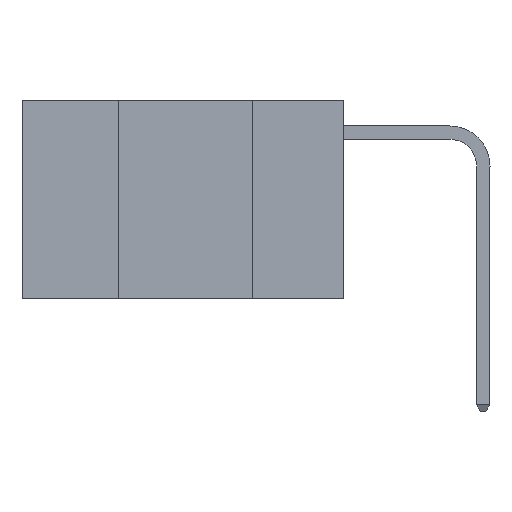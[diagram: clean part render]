
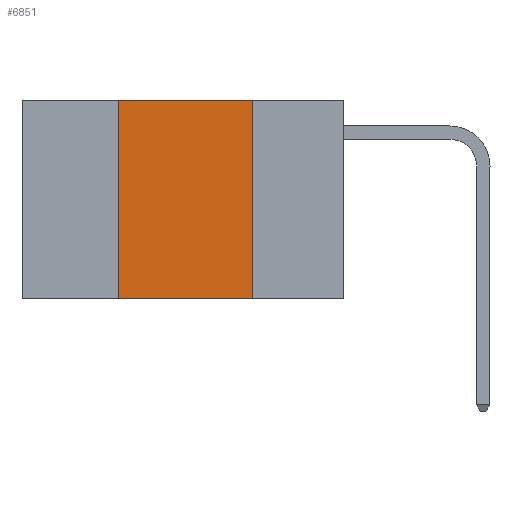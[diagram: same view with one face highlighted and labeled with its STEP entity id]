
A CAD part, left-side view. The second image highlights one B-rep face of the part: STEP entity #6851.
In plain terms, the highlighted planar face has unit normal (-1, 0, 0).
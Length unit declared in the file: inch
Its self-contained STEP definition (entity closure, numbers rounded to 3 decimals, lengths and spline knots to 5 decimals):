
#168 = VECTOR ( 'NONE', #7796, 39.37008 ) ;
#457 = CARTESIAN_POINT ( 'NONE',  ( 0., 0.17, 0. ) ) ;
#489 = ORIENTED_EDGE ( 'NONE', *, *, #13231, .F. ) ;
#883 = CARTESIAN_POINT ( 'NONE',  ( 0., 0.6, 0. ) ) ;
#902 = VERTEX_POINT ( 'NONE', #7395 ) ;
#962 = FACE_OUTER_BOUND ( 'NONE', #11207, .T. ) ;
#1337 = VECTOR ( 'NONE', #9512, 39.37008 ) ;
#1562 = VERTEX_POINT ( 'NONE', #9704 ) ;
#2855 = LINE ( 'NONE', #457, #9727 ) ;
#3279 = LINE ( 'NONE', #13469, #9341 ) ;
#3357 = VERTEX_POINT ( 'NONE', #3571 ) ;
#3571 = CARTESIAN_POINT ( 'NONE',  ( 0., 0.17, 0. ) ) ;
#3733 = DIRECTION ( 'NONE',  ( 0., -1., 0. ) ) ;
#5441 = CARTESIAN_POINT ( 'NONE',  ( 0., 0.42, 0. ) ) ;
#5551 = CARTESIAN_POINT ( 'NONE',  ( 0., 0.42, -0.37 ) ) ;
#6334 = DIRECTION ( 'NONE',  ( 0., 0., -1. ) ) ;
#6836 = LINE ( 'NONE', #5441, #168 ) ;
#6851 = ADVANCED_FACE ( 'NONE', ( #962 ), #11250, .F. ) ;
#7395 = CARTESIAN_POINT ( 'NONE',  ( 0., 0.42, 0. ) ) ;
#7500 = ORIENTED_EDGE ( 'NONE', *, *, #15976, .F. ) ;
#7796 = DIRECTION ( 'NONE',  ( 0., 0., 1. ) ) ;
#7878 = ORIENTED_EDGE ( 'NONE', *, *, #9794, .T. ) ;
#9135 = DIRECTION ( 'NONE',  ( 0., 0., -1. ) ) ;
#9341 = VECTOR ( 'NONE', #3733, 39.37008 ) ;
#9512 = DIRECTION ( 'NONE',  ( 0., -1., 0. ) ) ;
#9704 = CARTESIAN_POINT ( 'NONE',  ( 0., 0.17, -0.37 ) ) ;
#9727 = VECTOR ( 'NONE', #9135, 39.37008 ) ;
#9794 = EDGE_CURVE ( 'NONE', #15168, #1562, #3279, .T. ) ;
#11204 = LINE ( 'NONE', #883, #1337 ) ;
#11207 = EDGE_LOOP ( 'NONE', ( #12562, #7500, #489, #7878 ) ) ;
#11250 = PLANE ( 'NONE',  #12508 ) ;
#12490 = CARTESIAN_POINT ( 'NONE',  ( 0., 0.6, 0. ) ) ;
#12508 = AXIS2_PLACEMENT_3D ( 'NONE', #12490, #13752, #6334 ) ;
#12562 = ORIENTED_EDGE ( 'NONE', *, *, #13276, .F. ) ;
#13231 = EDGE_CURVE ( 'NONE', #15168, #902, #6836, .T. ) ;
#13276 = EDGE_CURVE ( 'NONE', #3357, #1562, #2855, .T. ) ;
#13469 = CARTESIAN_POINT ( 'NONE',  ( 0., 0.6, -0.37 ) ) ;
#13752 = DIRECTION ( 'NONE',  ( 1., 0., 0. ) ) ;
#15168 = VERTEX_POINT ( 'NONE', #5551 ) ;
#15976 = EDGE_CURVE ( 'NONE', #902, #3357, #11204, .T. ) ;
